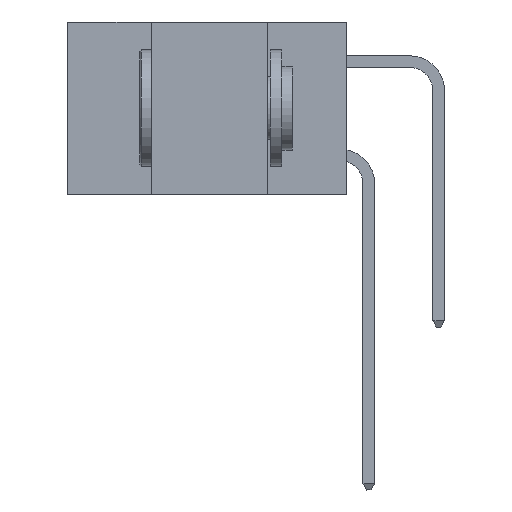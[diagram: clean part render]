
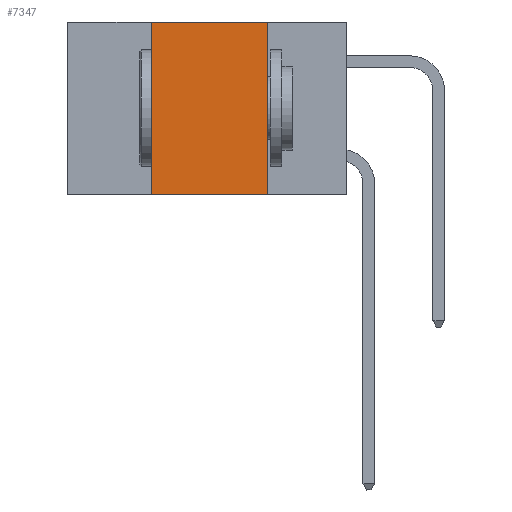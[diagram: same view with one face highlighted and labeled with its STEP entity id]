
A CAD part, left-side view. The second image highlights one B-rep face of the part: STEP entity #7347.
In plain terms, the highlighted planar face has unit normal (-1, 0, 0).
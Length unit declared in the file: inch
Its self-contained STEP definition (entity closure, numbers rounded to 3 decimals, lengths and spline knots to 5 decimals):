
#530 = DIRECTION ( 'NONE',  ( 0., -1., 0. ) ) ;
#1282 = VECTOR ( 'NONE', #4649, 39.37008 ) ;
#2505 = CARTESIAN_POINT ( 'NONE',  ( 0., 0.6, -0.37 ) ) ;
#3796 = EDGE_CURVE ( 'NONE', #22976, #23501, #24176, .T. ) ;
#3937 = LINE ( 'NONE', #2505, #11893 ) ;
#4649 = DIRECTION ( 'NONE',  ( 0., 0., 1. ) ) ;
#4736 = VECTOR ( 'NONE', #530, 39.37008 ) ;
#4799 = LINE ( 'NONE', #21586, #1282 ) ;
#4819 = CARTESIAN_POINT ( 'NONE',  ( 0., 0.42, -0.37 ) ) ;
#5355 = DIRECTION ( 'NONE',  ( 0., -1., 0. ) ) ;
#7347 = ADVANCED_FACE ( 'NONE', ( #29987 ), #35456, .F. ) ;
#9341 = CARTESIAN_POINT ( 'NONE',  ( 0., 0.17, 0. ) ) ;
#11387 = EDGE_CURVE ( 'NONE', #24791, #23501, #3937, .T. ) ;
#11893 = VECTOR ( 'NONE', #5355, 39.37008 ) ;
#12320 = DIRECTION ( 'NONE',  ( 0., 0., -1. ) ) ;
#13305 = EDGE_LOOP ( 'NONE', ( #16665, #30776, #35878, #33165 ) ) ;
#16551 = DIRECTION ( 'NONE',  ( 1., 0., 0. ) ) ;
#16665 = ORIENTED_EDGE ( 'NONE', *, *, #3796, .F. ) ;
#17465 = CARTESIAN_POINT ( 'NONE',  ( 0., 0.6, 0. ) ) ;
#18232 = VERTEX_POINT ( 'NONE', #35512 ) ;
#18555 = CARTESIAN_POINT ( 'NONE',  ( 0., 0.6, 0. ) ) ;
#20030 = CARTESIAN_POINT ( 'NONE',  ( 0., 0.17, 0. ) ) ;
#21586 = CARTESIAN_POINT ( 'NONE',  ( 0., 0.42, 0. ) ) ;
#22976 = VERTEX_POINT ( 'NONE', #20030 ) ;
#23302 = VECTOR ( 'NONE', #12320, 39.37008 ) ;
#23501 = VERTEX_POINT ( 'NONE', #32820 ) ;
#24176 = LINE ( 'NONE', #9341, #23302 ) ;
#24791 = VERTEX_POINT ( 'NONE', #4819 ) ;
#25197 = DIRECTION ( 'NONE',  ( 0., 0., -1. ) ) ;
#27318 = LINE ( 'NONE', #17465, #4736 ) ;
#29987 = FACE_OUTER_BOUND ( 'NONE', #13305, .T. ) ;
#30776 = ORIENTED_EDGE ( 'NONE', *, *, #31067, .F. ) ;
#31067 = EDGE_CURVE ( 'NONE', #18232, #22976, #27318, .T. ) ;
#31813 = EDGE_CURVE ( 'NONE', #24791, #18232, #4799, .T. ) ;
#32820 = CARTESIAN_POINT ( 'NONE',  ( 0., 0.17, -0.37 ) ) ;
#33165 = ORIENTED_EDGE ( 'NONE', *, *, #11387, .T. ) ;
#33999 = AXIS2_PLACEMENT_3D ( 'NONE', #18555, #16551, #25197 ) ;
#35456 = PLANE ( 'NONE',  #33999 ) ;
#35512 = CARTESIAN_POINT ( 'NONE',  ( 0., 0.42, 0. ) ) ;
#35878 = ORIENTED_EDGE ( 'NONE', *, *, #31813, .F. ) ;
